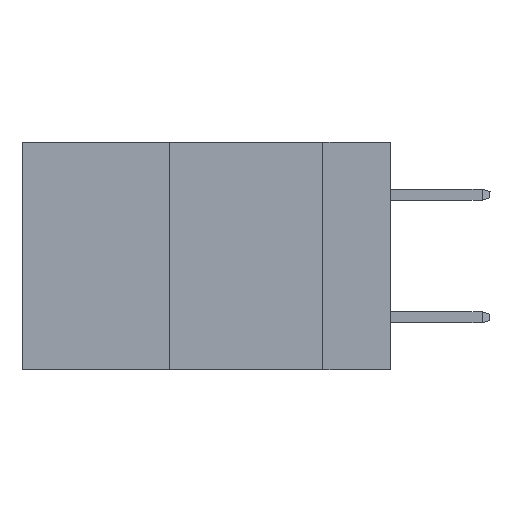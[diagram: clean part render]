
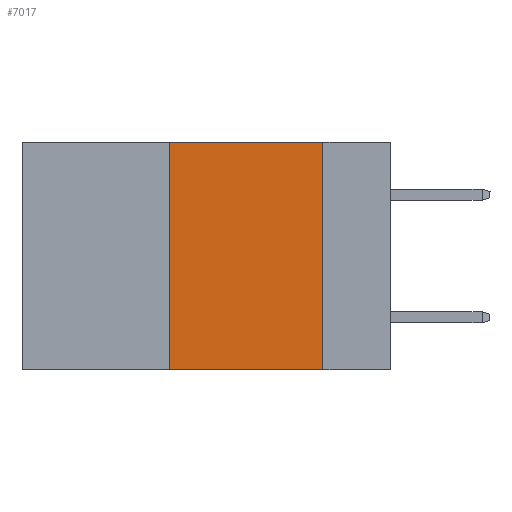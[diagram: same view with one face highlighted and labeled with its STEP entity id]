
A CAD part, left-side view. The second image highlights one B-rep face of the part: STEP entity #7017.
In plain terms, the highlighted planar face has unit normal (-1, 0, 0).
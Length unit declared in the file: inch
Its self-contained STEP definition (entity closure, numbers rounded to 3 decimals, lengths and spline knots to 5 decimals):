
#228 = ORIENTED_EDGE ( 'NONE', *, *, #9022, .F. ) ;
#559 = LINE ( 'NONE', #9993, #3558 ) ;
#633 = PLANE ( 'NONE',  #2712 ) ;
#688 = EDGE_CURVE ( 'NONE', #2587, #4324, #559, .T. ) ;
#1129 = LINE ( 'NONE', #8191, #2030 ) ;
#1610 = FACE_OUTER_BOUND ( 'NONE', #2017, .T. ) ;
#1911 = CARTESIAN_POINT ( 'NONE',  ( 0., 0.36, 0. ) ) ;
#2017 = EDGE_LOOP ( 'NONE', ( #3702, #4999, #228, #4882 ) ) ;
#2030 = VECTOR ( 'NONE', #4326, 39.37008 ) ;
#2330 = DIRECTION ( 'NONE',  ( 0., 0., -1. ) ) ;
#2587 = VERTEX_POINT ( 'NONE', #4491 ) ;
#2673 = LINE ( 'NONE', #1911, #5341 ) ;
#2712 = AXIS2_PLACEMENT_3D ( 'NONE', #2955, #6917, #2330 ) ;
#2947 = DIRECTION ( 'NONE',  ( 0., 0., -1. ) ) ;
#2955 = CARTESIAN_POINT ( 'NONE',  ( 0., 0.6, 0. ) ) ;
#3029 = CARTESIAN_POINT ( 'NONE',  ( 0., 0.36, 0. ) ) ;
#3558 = VECTOR ( 'NONE', #2947, 39.37008 ) ;
#3702 = ORIENTED_EDGE ( 'NONE', *, *, #688, .F. ) ;
#4324 = VERTEX_POINT ( 'NONE', #4479 ) ;
#4326 = DIRECTION ( 'NONE',  ( 0., -1., 0. ) ) ;
#4479 = CARTESIAN_POINT ( 'NONE',  ( 0., 0.11, -0.37 ) ) ;
#4491 = CARTESIAN_POINT ( 'NONE',  ( 0., 0.11, 0. ) ) ;
#4863 = DIRECTION ( 'NONE',  ( 0., -1., 0. ) ) ;
#4882 = ORIENTED_EDGE ( 'NONE', *, *, #7693, .T. ) ;
#4999 = ORIENTED_EDGE ( 'NONE', *, *, #9312, .F. ) ;
#5341 = VECTOR ( 'NONE', #5829, 39.37008 ) ;
#5363 = VECTOR ( 'NONE', #4863, 39.37008 ) ;
#5829 = DIRECTION ( 'NONE',  ( 0., 0., 1. ) ) ;
#6471 = CARTESIAN_POINT ( 'NONE',  ( 0., 0.36, -0.37 ) ) ;
#6917 = DIRECTION ( 'NONE',  ( 1., 0., 0. ) ) ;
#7017 = ADVANCED_FACE ( 'NONE', ( #1610 ), #633, .F. ) ;
#7693 = EDGE_CURVE ( 'NONE', #9749, #4324, #1129, .T. ) ;
#8191 = CARTESIAN_POINT ( 'NONE',  ( 0., 0.6, -0.37 ) ) ;
#8727 = LINE ( 'NONE', #9439, #5363 ) ;
#9022 = EDGE_CURVE ( 'NONE', #9749, #9215, #2673, .T. ) ;
#9215 = VERTEX_POINT ( 'NONE', #3029 ) ;
#9312 = EDGE_CURVE ( 'NONE', #9215, #2587, #8727, .T. ) ;
#9439 = CARTESIAN_POINT ( 'NONE',  ( 0., 0.6, 0. ) ) ;
#9749 = VERTEX_POINT ( 'NONE', #6471 ) ;
#9993 = CARTESIAN_POINT ( 'NONE',  ( 0., 0.11, 0. ) ) ;
